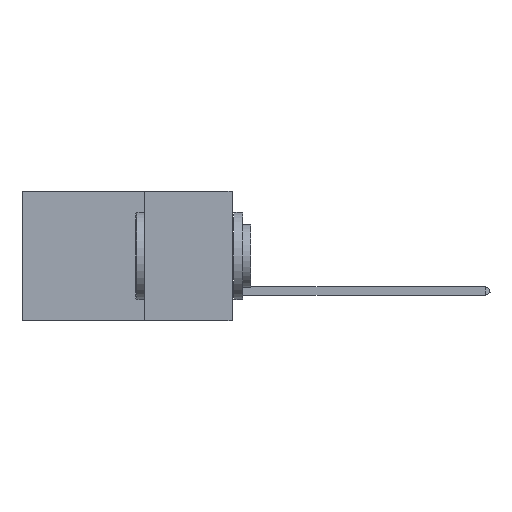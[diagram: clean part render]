
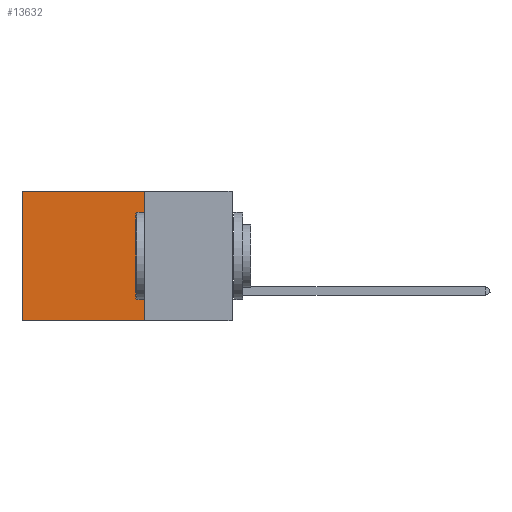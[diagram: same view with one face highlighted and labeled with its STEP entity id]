
A CAD part, left-side view. The second image highlights one B-rep face of the part: STEP entity #13632.
In plain terms, the highlighted planar face has unit normal (-1, 0, 0).
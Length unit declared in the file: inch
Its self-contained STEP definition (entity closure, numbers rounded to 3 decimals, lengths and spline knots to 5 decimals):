
#393 = EDGE_LOOP ( 'NONE', ( #10517, #5047, #6308, #11313 ) ) ;
#995 = VERTEX_POINT ( 'NONE', #9869 ) ;
#1042 = LINE ( 'NONE', #6743, #12620 ) ;
#1772 = CARTESIAN_POINT ( 'NONE',  ( 0.2875, 0.25, 0. ) ) ;
#1829 = DIRECTION ( 'NONE',  ( 0., 0., -1. ) ) ;
#1875 = DIRECTION ( 'NONE',  ( 0., 0., -1. ) ) ;
#2054 = LINE ( 'NONE', #1772, #14010 ) ;
#2403 = EDGE_CURVE ( 'NONE', #7686, #11604, #1042, .T. ) ;
#2579 = CARTESIAN_POINT ( 'NONE',  ( 0.2875, 0.25, 0. ) ) ;
#3531 = AXIS2_PLACEMENT_3D ( 'NONE', #2579, #13023, #1829 ) ;
#4104 = DIRECTION ( 'NONE',  ( 0., 1., 0. ) ) ;
#4936 = DIRECTION ( 'NONE',  ( 0., 1., 0. ) ) ;
#5047 = ORIENTED_EDGE ( 'NONE', *, *, #9469, .F. ) ;
#5183 = CARTESIAN_POINT ( 'NONE',  ( 0.2875, 0.6, -0.37 ) ) ;
#5244 = FACE_OUTER_BOUND ( 'NONE', #393, .T. ) ;
#6308 = ORIENTED_EDGE ( 'NONE', *, *, #7446, .F. ) ;
#6743 = CARTESIAN_POINT ( 'NONE',  ( 0.2875, 0.6, 0. ) ) ;
#7446 = EDGE_CURVE ( 'NONE', #995, #14089, #2054, .T. ) ;
#7686 = VERTEX_POINT ( 'NONE', #9142 ) ;
#7910 = DIRECTION ( 'NONE',  ( 0., 0., -1. ) ) ;
#8189 = LINE ( 'NONE', #12026, #12340 ) ;
#9142 = CARTESIAN_POINT ( 'NONE',  ( 0.2875, 0.6, 0. ) ) ;
#9172 = LINE ( 'NONE', #13553, #11150 ) ;
#9469 = EDGE_CURVE ( 'NONE', #14089, #11604, #9172, .T. ) ;
#9869 = CARTESIAN_POINT ( 'NONE',  ( 0.2875, 0.25, 0. ) ) ;
#10517 = ORIENTED_EDGE ( 'NONE', *, *, #2403, .T. ) ;
#10778 = PLANE ( 'NONE',  #3531 ) ;
#11150 = VECTOR ( 'NONE', #4104, 39.37008 ) ;
#11313 = ORIENTED_EDGE ( 'NONE', *, *, #12689, .T. ) ;
#11604 = VERTEX_POINT ( 'NONE', #5183 ) ;
#12026 = CARTESIAN_POINT ( 'NONE',  ( 0.2875, 0.25, 0. ) ) ;
#12318 = CARTESIAN_POINT ( 'NONE',  ( 0.2875, 0.25, -0.37 ) ) ;
#12340 = VECTOR ( 'NONE', #4936, 39.37008 ) ;
#12620 = VECTOR ( 'NONE', #7910, 39.37008 ) ;
#12689 = EDGE_CURVE ( 'NONE', #995, #7686, #8189, .T. ) ;
#13023 = DIRECTION ( 'NONE',  ( 1., 0., 0. ) ) ;
#13553 = CARTESIAN_POINT ( 'NONE',  ( 0.2875, 0.25, -0.37 ) ) ;
#13632 = ADVANCED_FACE ( 'NONE', ( #5244 ), #10778, .F. ) ;
#14010 = VECTOR ( 'NONE', #1875, 39.37008 ) ;
#14089 = VERTEX_POINT ( 'NONE', #12318 ) ;
